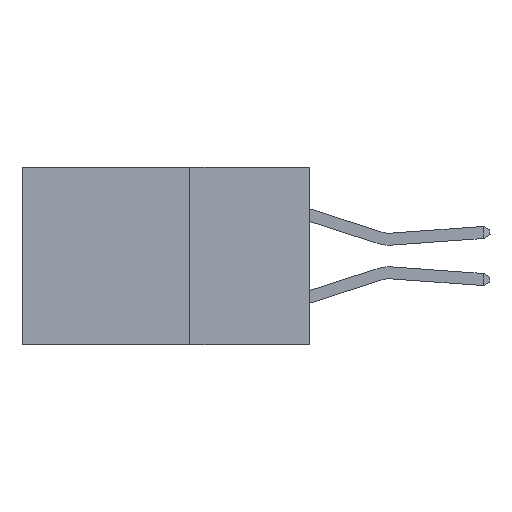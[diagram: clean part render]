
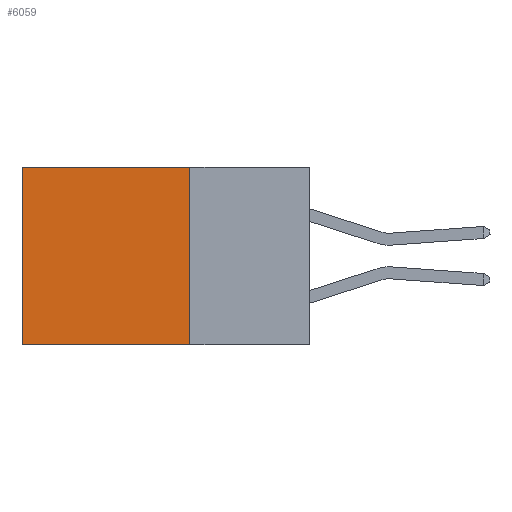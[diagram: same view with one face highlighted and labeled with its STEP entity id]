
A CAD part, left-side view. The second image highlights one B-rep face of the part: STEP entity #6059.
In plain terms, the highlighted planar face has unit normal (-1, 0, 0).
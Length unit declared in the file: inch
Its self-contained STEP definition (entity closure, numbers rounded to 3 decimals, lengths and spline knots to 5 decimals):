
#170 = DIRECTION ( 'NONE',  ( 0., 0., -1. ) ) ;
#476 = EDGE_CURVE ( 'NONE', #2450, #7915, #11679, .T. ) ;
#566 = VERTEX_POINT ( 'NONE', #11247 ) ;
#732 = LINE ( 'NONE', #11148, #4993 ) ;
#799 = VECTOR ( 'NONE', #4081, 39.37008 ) ;
#1101 = LINE ( 'NONE', #4073, #799 ) ;
#1676 = FACE_OUTER_BOUND ( 'NONE', #1934, .T. ) ;
#1934 = EDGE_LOOP ( 'NONE', ( #10472, #3928, #9988, #8479 ) ) ;
#2323 = VERTEX_POINT ( 'NONE', #8923 ) ;
#2450 = VERTEX_POINT ( 'NONE', #6695 ) ;
#2732 = CARTESIAN_POINT ( 'NONE',  ( 0.2615, 0.25, 0. ) ) ;
#3333 = AXIS2_PLACEMENT_3D ( 'NONE', #6643, #6470, #6449 ) ;
#3928 = ORIENTED_EDGE ( 'NONE', *, *, #9098, .F. ) ;
#4072 = CARTESIAN_POINT ( 'NONE',  ( 0.2615, 0.6, 0. ) ) ;
#4073 = CARTESIAN_POINT ( 'NONE',  ( 0.2615, 0.6, -0.37 ) ) ;
#4081 = DIRECTION ( 'NONE',  ( 0., 0., -1. ) ) ;
#4129 = LINE ( 'NONE', #5643, #8985 ) ;
#4415 = VECTOR ( 'NONE', #9218, 39.37008 ) ;
#4732 = DIRECTION ( 'NONE',  ( 0., 1., 0. ) ) ;
#4993 = VECTOR ( 'NONE', #4732, 39.37008 ) ;
#5643 = CARTESIAN_POINT ( 'NONE',  ( 0.2615, 0.25, -0.37 ) ) ;
#6059 = ADVANCED_FACE ( 'NONE', ( #1676 ), #6570, .F. ) ;
#6364 = EDGE_CURVE ( 'NONE', #7915, #2323, #1101, .T. ) ;
#6449 = DIRECTION ( 'NONE',  ( 0., 0., -1. ) ) ;
#6470 = DIRECTION ( 'NONE',  ( 1., 0., 0. ) ) ;
#6570 = PLANE ( 'NONE',  #3333 ) ;
#6643 = CARTESIAN_POINT ( 'NONE',  ( 0.2615, 0.25, -0.37 ) ) ;
#6695 = CARTESIAN_POINT ( 'NONE',  ( 0.2615, 0.25, 0. ) ) ;
#7915 = VERTEX_POINT ( 'NONE', #4072 ) ;
#8479 = ORIENTED_EDGE ( 'NONE', *, *, #476, .T. ) ;
#8923 = CARTESIAN_POINT ( 'NONE',  ( 0.2615, 0.6, -0.37 ) ) ;
#8985 = VECTOR ( 'NONE', #170, 39.37008 ) ;
#9098 = EDGE_CURVE ( 'NONE', #566, #2323, #732, .T. ) ;
#9218 = DIRECTION ( 'NONE',  ( 0., 1., 0. ) ) ;
#9988 = ORIENTED_EDGE ( 'NONE', *, *, #11660, .F. ) ;
#10472 = ORIENTED_EDGE ( 'NONE', *, *, #6364, .T. ) ;
#11148 = CARTESIAN_POINT ( 'NONE',  ( 0.2615, 0.25, -0.37 ) ) ;
#11247 = CARTESIAN_POINT ( 'NONE',  ( 0.2615, 0.25, -0.37 ) ) ;
#11660 = EDGE_CURVE ( 'NONE', #2450, #566, #4129, .T. ) ;
#11679 = LINE ( 'NONE', #2732, #4415 ) ;
